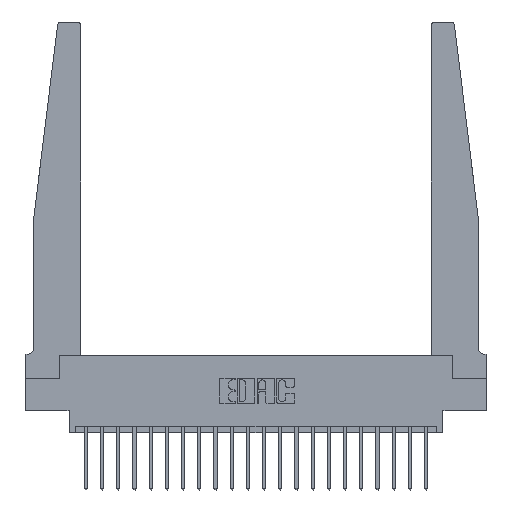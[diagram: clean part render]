
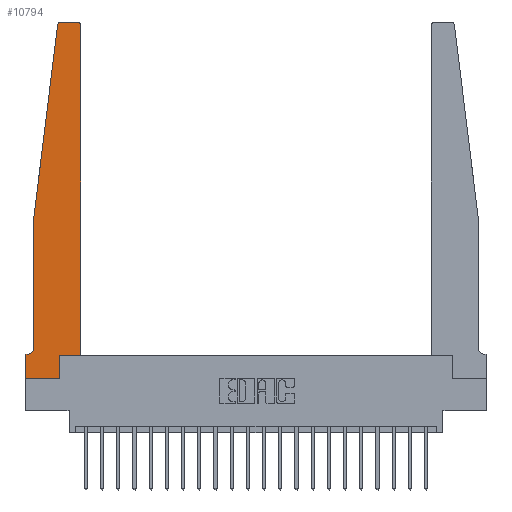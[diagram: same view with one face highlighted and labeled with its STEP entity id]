
A CAD part, top view. The second image highlights one B-rep face of the part: STEP entity #10794.
In plain terms, the highlighted planar face has unit normal (0, 0, 1).
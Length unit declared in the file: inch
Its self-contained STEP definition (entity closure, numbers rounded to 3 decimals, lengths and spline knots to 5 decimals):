
#96 = CARTESIAN_POINT ( 'NONE',  ( 0.395, 2.72, 0.37 ) ) ;
#859 = ORIENTED_EDGE ( 'NONE', *, *, #13294, .T. ) ;
#893 = LINE ( 'NONE', #12889, #10279 ) ;
#1070 = DIRECTION ( 'NONE',  ( 0., -1., 0. ) ) ;
#1185 = FACE_OUTER_BOUND ( 'NONE', #22106, .T. ) ;
#1309 = CARTESIAN_POINT ( 'NONE',  ( 0.425, 0.18, 0.37 ) ) ;
#1911 = DIRECTION ( 'NONE',  ( 0., 0., -1. ) ) ;
#1922 = EDGE_CURVE ( 'NONE', #22347, #17789, #18554, .T. ) ;
#2083 = EDGE_CURVE ( 'NONE', #17789, #15115, #6749, .T. ) ;
#2156 = DIRECTION ( 'NONE',  ( 1., 0., 0. ) ) ;
#2365 = CARTESIAN_POINT ( 'NONE',  ( 0.015, 0.1875, 0.37 ) ) ;
#2639 = VERTEX_POINT ( 'NONE', #7203 ) ;
#2704 = DIRECTION ( 'NONE',  ( -1., 0., 0. ) ) ;
#2769 = AXIS2_PLACEMENT_3D ( 'NONE', #17206, #1911, #20979 ) ;
#2946 = ORIENTED_EDGE ( 'NONE', *, *, #20350, .T. ) ;
#2949 = CARTESIAN_POINT ( 'NONE',  ( 0.425, 0.18, 0.37 ) ) ;
#3255 = CARTESIAN_POINT ( 'NONE',  ( 0., 0.1875, 0.37 ) ) ;
#3743 = VECTOR ( 'NONE', #9372, 39.37008 ) ;
#3876 = CIRCLE ( 'NONE', #2769, 0.05 ) ;
#4482 = PLANE ( 'NONE',  #14498 ) ;
#4569 = ORIENTED_EDGE ( 'NONE', *, *, #1922, .T. ) ;
#4600 = CARTESIAN_POINT ( 'NONE',  ( 0., 0.1875, 0.37 ) ) ;
#4802 = CARTESIAN_POINT ( 'NONE',  ( 0.065, 1.25, 0.37 ) ) ;
#5027 = LINE ( 'NONE', #11928, #13867 ) ;
#5284 = ORIENTED_EDGE ( 'NONE', *, *, #13074, .T. ) ;
#5839 = ORIENTED_EDGE ( 'NONE', *, *, #8218, .T. ) ;
#5954 = ORIENTED_EDGE ( 'NONE', *, *, #11893, .T. ) ;
#6174 = DIRECTION ( 'NONE',  ( 1., 0., 0. ) ) ;
#6182 = LINE ( 'NONE', #20026, #6853 ) ;
#6220 = DIRECTION ( 'NONE',  ( 0., 1., 0. ) ) ;
#6463 = EDGE_CURVE ( 'NONE', #14047, #20238, #6182, .T. ) ;
#6484 = LINE ( 'NONE', #4802, #19670 ) ;
#6585 = LINE ( 'NONE', #21819, #9159 ) ;
#6700 = DIRECTION ( 'NONE',  ( 1., 0., 0. ) ) ;
#6749 = CIRCLE ( 'NONE', #18683, 0.03 ) ;
#6853 = VECTOR ( 'NONE', #8002, 39.37008 ) ;
#7203 = CARTESIAN_POINT ( 'NONE',  ( 0.2605, 0.18, 0.37 ) ) ;
#8002 = DIRECTION ( 'NONE',  ( 0., -1., 0. ) ) ;
#8096 = DIRECTION ( 'NONE',  ( 1., 0., 0. ) ) ;
#8157 = CARTESIAN_POINT ( 'NONE',  ( 0., 0., 0.37 ) ) ;
#8218 = EDGE_CURVE ( 'NONE', #9929, #19687, #16527, .T. ) ;
#8897 = EDGE_CURVE ( 'NONE', #15115, #9929, #893, .T. ) ;
#8910 = VERTEX_POINT ( 'NONE', #21422 ) ;
#9159 = VECTOR ( 'NONE', #1070, 39.37008 ) ;
#9275 = CARTESIAN_POINT ( 'NONE',  ( 0.065, 1.25, 0.37 ) ) ;
#9326 = CARTESIAN_POINT ( 'NONE',  ( 0.24675, 2.72367, 0.37 ) ) ;
#9372 = DIRECTION ( 'NONE',  ( -1., 0., 0. ) ) ;
#9440 = CARTESIAN_POINT ( 'NONE',  ( 0.2605, 0.18, 0.37 ) ) ;
#9929 = VERTEX_POINT ( 'NONE', #16201 ) ;
#10103 = CARTESIAN_POINT ( 'NONE',  ( 0.27653, 2.72, 0.37 ) ) ;
#10274 = DIRECTION ( 'NONE',  ( 0., 0., 1. ) ) ;
#10279 = VECTOR ( 'NONE', #2704, 39.37008 ) ;
#10617 = VECTOR ( 'NONE', #14739, 39.37008 ) ;
#10794 = ADVANCED_FACE ( 'NONE', ( #1185 ), #4482, .T. ) ;
#11185 = LINE ( 'NONE', #21297, #3743 ) ;
#11761 = ORIENTED_EDGE ( 'NONE', *, *, #22127, .T. ) ;
#11893 = EDGE_CURVE ( 'NONE', #15300, #14047, #11185, .T. ) ;
#11928 = CARTESIAN_POINT ( 'NONE',  ( 0., 0., 0.37 ) ) ;
#12889 = CARTESIAN_POINT ( 'NONE',  ( 0.25, 2.75, 0.37 ) ) ;
#13074 = EDGE_CURVE ( 'NONE', #19834, #2639, #17835, .T. ) ;
#13168 = DIRECTION ( 'NONE',  ( 0., 0., 1. ) ) ;
#13179 = EDGE_CURVE ( 'NONE', #16503, #8910, #6585, .T. ) ;
#13259 = EDGE_CURVE ( 'NONE', #19687, #16503, #6484, .T. ) ;
#13294 = EDGE_CURVE ( 'NONE', #20238, #19834, #5027, .T. ) ;
#13393 = DIRECTION ( 'NONE',  ( 0., 0., 1. ) ) ;
#13607 = CARTESIAN_POINT ( 'NONE',  ( 0.2605, 0., 0.37 ) ) ;
#13867 = VECTOR ( 'NONE', #2156, 39.37008 ) ;
#14030 = VECTOR ( 'NONE', #6174, 39.37008 ) ;
#14047 = VERTEX_POINT ( 'NONE', #3255 ) ;
#14498 = AXIS2_PLACEMENT_3D ( 'NONE', #4600, #13168, #8096 ) ;
#14533 = ORIENTED_EDGE ( 'NONE', *, *, #6463, .T. ) ;
#14542 = ORIENTED_EDGE ( 'NONE', *, *, #8897, .T. ) ;
#14739 = DIRECTION ( 'NONE',  ( 0., 1., 0. ) ) ;
#14979 = LINE ( 'NONE', #1309, #14030 ) ;
#15115 = VERTEX_POINT ( 'NONE', #15491 ) ;
#15199 = ORIENTED_EDGE ( 'NONE', *, *, #2083, .T. ) ;
#15300 = VERTEX_POINT ( 'NONE', #2365 ) ;
#15447 = CARTESIAN_POINT ( 'NONE',  ( 0.425, 2.72, 0.37 ) ) ;
#15491 = CARTESIAN_POINT ( 'NONE',  ( 0.395, 2.75, 0.37 ) ) ;
#16201 = CARTESIAN_POINT ( 'NONE',  ( 0.27653, 2.75, 0.37 ) ) ;
#16503 = VERTEX_POINT ( 'NONE', #9275 ) ;
#16527 = CIRCLE ( 'NONE', #19406, 0.03 ) ;
#17193 = DIRECTION ( 'NONE',  ( 1., 0., 0. ) ) ;
#17206 = CARTESIAN_POINT ( 'NONE',  ( 0.015, 0.2375, 0.37 ) ) ;
#17789 = VERTEX_POINT ( 'NONE', #15447 ) ;
#17835 = LINE ( 'NONE', #9440, #10617 ) ;
#18232 = ORIENTED_EDGE ( 'NONE', *, *, #13259, .T. ) ;
#18385 = DIRECTION ( 'NONE',  ( -0.122, -0.992, 0. ) ) ;
#18554 = LINE ( 'NONE', #2949, #21253 ) ;
#18683 = AXIS2_PLACEMENT_3D ( 'NONE', #96, #10274, #17193 ) ;
#18838 = CARTESIAN_POINT ( 'NONE',  ( 0.425, 0.18, 0.37 ) ) ;
#19406 = AXIS2_PLACEMENT_3D ( 'NONE', #10103, #13393, #6700 ) ;
#19670 = VECTOR ( 'NONE', #18385, 39.37008 ) ;
#19687 = VERTEX_POINT ( 'NONE', #9326 ) ;
#19834 = VERTEX_POINT ( 'NONE', #13607 ) ;
#20026 = CARTESIAN_POINT ( 'NONE',  ( 0., 0., 0.37 ) ) ;
#20238 = VERTEX_POINT ( 'NONE', #8157 ) ;
#20350 = EDGE_CURVE ( 'NONE', #8910, #15300, #3876, .T. ) ;
#20979 = DIRECTION ( 'NONE',  ( -1., 0., 0. ) ) ;
#21253 = VECTOR ( 'NONE', #6220, 39.37008 ) ;
#21297 = CARTESIAN_POINT ( 'NONE',  ( 0.065, 0.1875, 0.37 ) ) ;
#21422 = CARTESIAN_POINT ( 'NONE',  ( 0.065, 0.2375, 0.37 ) ) ;
#21819 = CARTESIAN_POINT ( 'NONE',  ( 0.065, 1.25, 0.37 ) ) ;
#22106 = EDGE_LOOP ( 'NONE', ( #14542, #5839, #18232, #22291, #2946, #5954, #14533, #859, #5284, #11761, #4569, #15199 ) ) ;
#22127 = EDGE_CURVE ( 'NONE', #2639, #22347, #14979, .T. ) ;
#22291 = ORIENTED_EDGE ( 'NONE', *, *, #13179, .T. ) ;
#22347 = VERTEX_POINT ( 'NONE', #18838 ) ;
